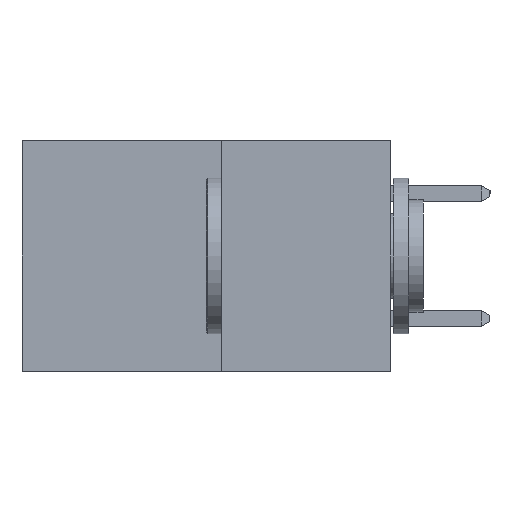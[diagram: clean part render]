
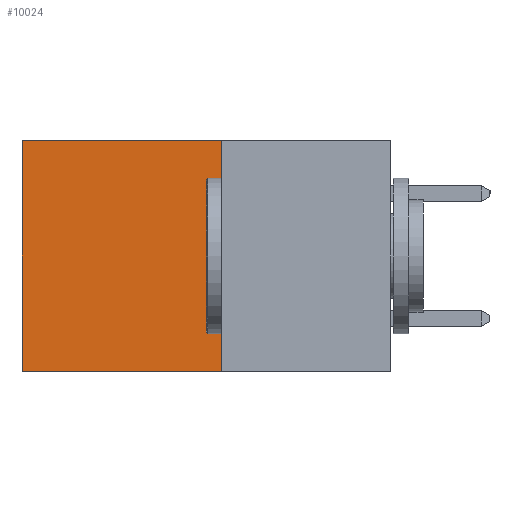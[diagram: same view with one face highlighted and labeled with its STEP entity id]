
A CAD part, left-side view. The second image highlights one B-rep face of the part: STEP entity #10024.
In plain terms, the highlighted planar face has unit normal (-1, 0, 0).
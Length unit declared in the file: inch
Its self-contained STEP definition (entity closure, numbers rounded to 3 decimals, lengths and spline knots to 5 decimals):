
#36 = CARTESIAN_POINT ( 'NONE',  ( 0.277, 0.59, 0. ) ) ;
#348 = DIRECTION ( 'NONE',  ( 1., 0., 0. ) ) ;
#544 = VERTEX_POINT ( 'NONE', #7357 ) ;
#1511 = VERTEX_POINT ( 'NONE', #4903 ) ;
#1729 = DIRECTION ( 'NONE',  ( 0., 0., -1. ) ) ;
#1927 = EDGE_CURVE ( 'NONE', #7223, #5246, #2954, .T. ) ;
#2119 = CARTESIAN_POINT ( 'NONE',  ( 0.277, 0.59, -0.37 ) ) ;
#2954 = LINE ( 'NONE', #2119, #4852 ) ;
#3667 = VECTOR ( 'NONE', #8835, 39.37008 ) ;
#3739 = ORIENTED_EDGE ( 'NONE', *, *, #4970, .F. ) ;
#3821 = CARTESIAN_POINT ( 'NONE',  ( 0.277, 0.27, -0.37 ) ) ;
#4423 = PLANE ( 'NONE',  #5996 ) ;
#4516 = EDGE_LOOP ( 'NONE', ( #5542, #6992, #3739, #6437 ) ) ;
#4832 = DIRECTION ( 'NONE',  ( 0., 1., 0. ) ) ;
#4852 = VECTOR ( 'NONE', #1729, 39.37008 ) ;
#4903 = CARTESIAN_POINT ( 'NONE',  ( 0.277, 0.27, -0.37 ) ) ;
#4970 = EDGE_CURVE ( 'NONE', #544, #1511, #5748, .T. ) ;
#5146 = VECTOR ( 'NONE', #7539, 39.37008 ) ;
#5246 = VERTEX_POINT ( 'NONE', #8553 ) ;
#5327 = EDGE_CURVE ( 'NONE', #544, #7223, #6713, .T. ) ;
#5542 = ORIENTED_EDGE ( 'NONE', *, *, #1927, .T. ) ;
#5748 = LINE ( 'NONE', #9889, #3667 ) ;
#5962 = DIRECTION ( 'NONE',  ( 0., 0., -1. ) ) ;
#5996 = AXIS2_PLACEMENT_3D ( 'NONE', #9716, #348, #5962 ) ;
#6218 = EDGE_CURVE ( 'NONE', #1511, #5246, #6303, .T. ) ;
#6236 = FACE_OUTER_BOUND ( 'NONE', #4516, .T. ) ;
#6303 = LINE ( 'NONE', #3821, #7843 ) ;
#6437 = ORIENTED_EDGE ( 'NONE', *, *, #5327, .T. ) ;
#6713 = LINE ( 'NONE', #7530, #5146 ) ;
#6992 = ORIENTED_EDGE ( 'NONE', *, *, #6218, .F. ) ;
#7223 = VERTEX_POINT ( 'NONE', #36 ) ;
#7357 = CARTESIAN_POINT ( 'NONE',  ( 0.277, 0.27, 0. ) ) ;
#7530 = CARTESIAN_POINT ( 'NONE',  ( 0.277, 0.27, 0. ) ) ;
#7539 = DIRECTION ( 'NONE',  ( 0., 1., 0. ) ) ;
#7843 = VECTOR ( 'NONE', #4832, 39.37008 ) ;
#8553 = CARTESIAN_POINT ( 'NONE',  ( 0.277, 0.59, -0.37 ) ) ;
#8835 = DIRECTION ( 'NONE',  ( 0., 0., -1. ) ) ;
#9716 = CARTESIAN_POINT ( 'NONE',  ( 0.277, 0.27, -0.37 ) ) ;
#9889 = CARTESIAN_POINT ( 'NONE',  ( 0.277, 0.27, -0.37 ) ) ;
#10024 = ADVANCED_FACE ( 'NONE', ( #6236 ), #4423, .F. ) ;
